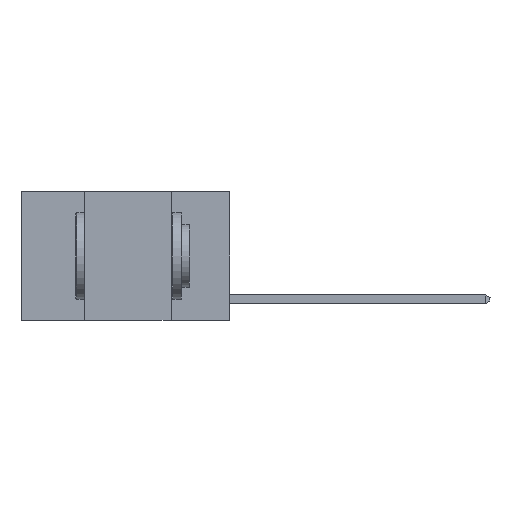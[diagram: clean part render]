
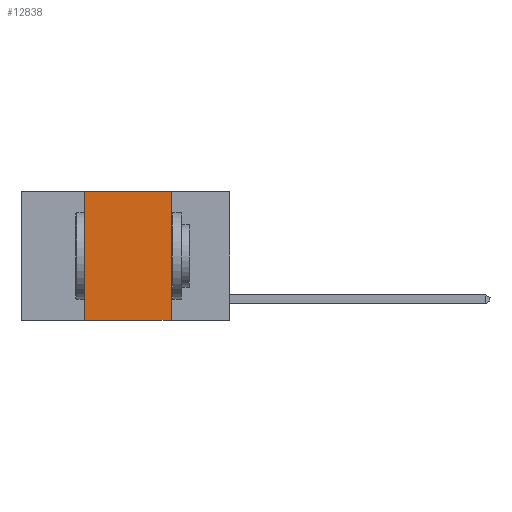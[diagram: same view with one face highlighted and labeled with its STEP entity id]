
A CAD part, left-side view. The second image highlights one B-rep face of the part: STEP entity #12838.
In plain terms, the highlighted planar face has unit normal (-1, 0, 0).
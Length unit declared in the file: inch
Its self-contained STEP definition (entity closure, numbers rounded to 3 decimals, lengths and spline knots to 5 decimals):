
#814 = DIRECTION ( 'NONE',  ( 0., 0., 1. ) ) ;
#3006 = AXIS2_PLACEMENT_3D ( 'NONE', #10656, #29004, #8389 ) ;
#4071 = DIRECTION ( 'NONE',  ( 0., 0., -1. ) ) ;
#4803 = ORIENTED_EDGE ( 'NONE', *, *, #17939, .F. ) ;
#6917 = VERTEX_POINT ( 'NONE', #27212 ) ;
#8389 = DIRECTION ( 'NONE',  ( 0., 0., -1. ) ) ;
#9230 = LINE ( 'NONE', #18420, #21303 ) ;
#10656 = CARTESIAN_POINT ( 'NONE',  ( 0., 0.6, 0. ) ) ;
#11192 = VERTEX_POINT ( 'NONE', #16220 ) ;
#11196 = VECTOR ( 'NONE', #4071, 39.37008 ) ;
#11454 = VECTOR ( 'NONE', #814, 39.37008 ) ;
#12548 = EDGE_CURVE ( 'NONE', #6917, #18472, #15524, .T. ) ;
#12838 = ADVANCED_FACE ( 'NONE', ( #17155 ), #26590, .F. ) ;
#13499 = EDGE_LOOP ( 'NONE', ( #15209, #18203, #4803, #25471 ) ) ;
#13553 = LINE ( 'NONE', #25274, #28839 ) ;
#13847 = DIRECTION ( 'NONE',  ( 0., -1., 0. ) ) ;
#14390 = CARTESIAN_POINT ( 'NONE',  ( 0., 0.42, 0. ) ) ;
#14672 = CARTESIAN_POINT ( 'NONE',  ( 0., 0.42, 0. ) ) ;
#15209 = ORIENTED_EDGE ( 'NONE', *, *, #12548, .F. ) ;
#15524 = LINE ( 'NONE', #24677, #11196 ) ;
#16220 = CARTESIAN_POINT ( 'NONE',  ( 0., 0.42, -0.37 ) ) ;
#17059 = CARTESIAN_POINT ( 'NONE',  ( 0., 0.17, -0.37 ) ) ;
#17155 = FACE_OUTER_BOUND ( 'NONE', #13499, .T. ) ;
#17939 = EDGE_CURVE ( 'NONE', #11192, #27152, #23683, .T. ) ;
#18203 = ORIENTED_EDGE ( 'NONE', *, *, #20075, .F. ) ;
#18420 = CARTESIAN_POINT ( 'NONE',  ( 0., 0.6, -0.37 ) ) ;
#18472 = VERTEX_POINT ( 'NONE', #17059 ) ;
#20075 = EDGE_CURVE ( 'NONE', #27152, #6917, #13553, .T. ) ;
#21303 = VECTOR ( 'NONE', #27578, 39.37008 ) ;
#23683 = LINE ( 'NONE', #14672, #11454 ) ;
#24677 = CARTESIAN_POINT ( 'NONE',  ( 0., 0.17, 0. ) ) ;
#24691 = EDGE_CURVE ( 'NONE', #11192, #18472, #9230, .T. ) ;
#25274 = CARTESIAN_POINT ( 'NONE',  ( 0., 0.6, 0. ) ) ;
#25471 = ORIENTED_EDGE ( 'NONE', *, *, #24691, .T. ) ;
#26590 = PLANE ( 'NONE',  #3006 ) ;
#27152 = VERTEX_POINT ( 'NONE', #14390 ) ;
#27212 = CARTESIAN_POINT ( 'NONE',  ( 0., 0.17, 0. ) ) ;
#27578 = DIRECTION ( 'NONE',  ( 0., -1., 0. ) ) ;
#28839 = VECTOR ( 'NONE', #13847, 39.37008 ) ;
#29004 = DIRECTION ( 'NONE',  ( 1., 0., 0. ) ) ;
